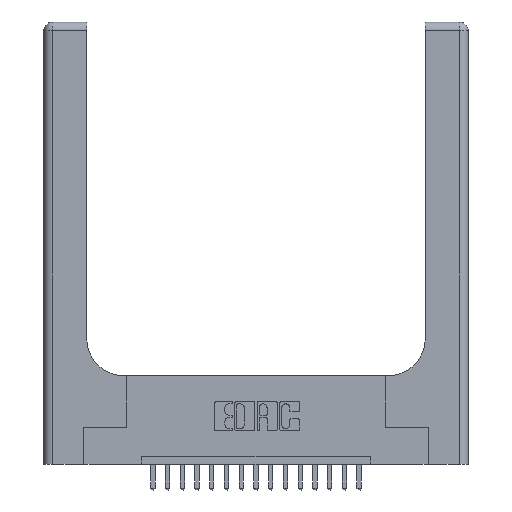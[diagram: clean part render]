
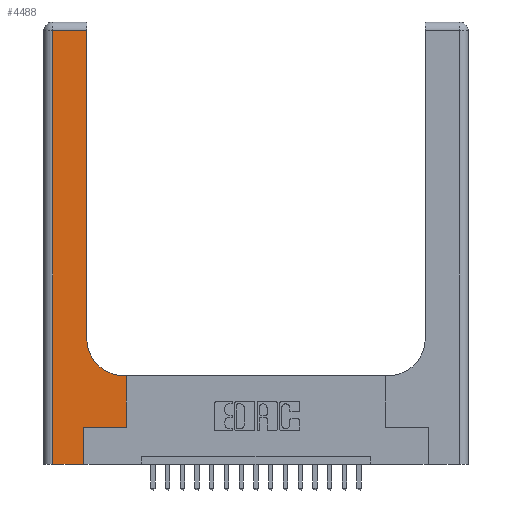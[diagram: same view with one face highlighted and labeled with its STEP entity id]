
A CAD part, top view. The second image highlights one B-rep face of the part: STEP entity #4488.
In plain terms, the highlighted planar face has unit normal (0, 0, 1).
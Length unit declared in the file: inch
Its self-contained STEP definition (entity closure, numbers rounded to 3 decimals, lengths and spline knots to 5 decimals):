
#148 = VECTOR ( 'NONE', #15924, 39.37008 ) ;
#211 = EDGE_CURVE ( 'NONE', #18725, #6965, #633, .T. ) ;
#633 = LINE ( 'NONE', #6570, #148 ) ;
#1206 = VERTEX_POINT ( 'NONE', #12824 ) ;
#1649 = VECTOR ( 'NONE', #11076, 39.37008 ) ;
#2056 = VECTOR ( 'NONE', #4676, 39.37008 ) ;
#2219 = EDGE_CURVE ( 'NONE', #10617, #5657, #18278, .T. ) ;
#2421 = CARTESIAN_POINT ( 'NONE',  ( 0.06, 0., 0.37 ) ) ;
#2588 = EDGE_CURVE ( 'NONE', #5657, #9849, #15346, .T. ) ;
#2597 = LINE ( 'NONE', #2917, #17723 ) ;
#2634 = VECTOR ( 'NONE', #16668, 39.37008 ) ;
#2917 = CARTESIAN_POINT ( 'NONE',  ( 0.2915, 0.6, 0.37 ) ) ;
#3111 = CARTESIAN_POINT ( 'NONE',  ( 0.269, 0., 0.37 ) ) ;
#3171 = DIRECTION ( 'NONE',  ( 0., 1., 0. ) ) ;
#3302 = EDGE_CURVE ( 'NONE', #10700, #18588, #15554, .T. ) ;
#3770 = LINE ( 'NONE', #3111, #2056 ) ;
#4225 = CARTESIAN_POINT ( 'NONE',  ( 0.269, 0., 0.37 ) ) ;
#4488 = ADVANCED_FACE ( 'NONE', ( #12314 ), #6179, .F. ) ;
#4625 = AXIS2_PLACEMENT_3D ( 'NONE', #11066, #9435, #5221 ) ;
#4671 = CARTESIAN_POINT ( 'NONE',  ( 0.5585, 0.6, 0.37 ) ) ;
#4676 = DIRECTION ( 'NONE',  ( 0., 1., 0. ) ) ;
#5146 = VERTEX_POINT ( 'NONE', #10031 ) ;
#5206 = ORIENTED_EDGE ( 'NONE', *, *, #19410, .T. ) ;
#5221 = DIRECTION ( 'NONE',  ( -1., 0., 0. ) ) ;
#5657 = VERTEX_POINT ( 'NONE', #7869 ) ;
#6179 = PLANE ( 'NONE',  #4625 ) ;
#6570 = CARTESIAN_POINT ( 'NONE',  ( 0., 2.94, 0.37 ) ) ;
#6953 = DIRECTION ( 'NONE',  ( 0., 1., 0. ) ) ;
#6965 = VERTEX_POINT ( 'NONE', #12682 ) ;
#7240 = VECTOR ( 'NONE', #10595, 39.37008 ) ;
#7242 = DIRECTION ( 'NONE',  ( 1., 0., 0. ) ) ;
#7333 = ORIENTED_EDGE ( 'NONE', *, *, #15643, .T. ) ;
#7588 = CIRCLE ( 'NONE', #10735, 0.25 ) ;
#7869 = CARTESIAN_POINT ( 'NONE',  ( 0.5585, 0.25, 0.37 ) ) ;
#7982 = DIRECTION ( 'NONE',  ( -1., 0., 0. ) ) ;
#8212 = CARTESIAN_POINT ( 'NONE',  ( 0.06, 3., 0.37 ) ) ;
#8257 = EDGE_CURVE ( 'NONE', #9849, #1206, #2597, .T. ) ;
#8568 = VECTOR ( 'NONE', #3171, 39.37008 ) ;
#9435 = DIRECTION ( 'NONE',  ( 0., 0., -1. ) ) ;
#9482 = CARTESIAN_POINT ( 'NONE',  ( 0.2915, 3., 0.37 ) ) ;
#9849 = VERTEX_POINT ( 'NONE', #4671 ) ;
#10031 = CARTESIAN_POINT ( 'NONE',  ( 0.2915, 0.85, 0.37 ) ) ;
#10049 = ORIENTED_EDGE ( 'NONE', *, *, #12741, .T. ) ;
#10530 = CARTESIAN_POINT ( 'NONE',  ( 0.2915, 2.94, 0.37 ) ) ;
#10595 = DIRECTION ( 'NONE',  ( 1., 0., 0. ) ) ;
#10617 = VERTEX_POINT ( 'NONE', #12881 ) ;
#10700 = VERTEX_POINT ( 'NONE', #2421 ) ;
#10735 = AXIS2_PLACEMENT_3D ( 'NONE', #16594, #19798, #7242 ) ;
#11066 = CARTESIAN_POINT ( 'NONE',  ( 0., 3., 0.37 ) ) ;
#11076 = DIRECTION ( 'NONE',  ( 0., -1., 0. ) ) ;
#12314 = FACE_OUTER_BOUND ( 'NONE', #19108, .T. ) ;
#12682 = CARTESIAN_POINT ( 'NONE',  ( 0.06, 2.94, 0.37 ) ) ;
#12741 = EDGE_CURVE ( 'NONE', #1206, #5146, #7588, .T. ) ;
#12824 = CARTESIAN_POINT ( 'NONE',  ( 0.5415, 0.6, 0.37 ) ) ;
#12881 = CARTESIAN_POINT ( 'NONE',  ( 0.269, 0.25, 0.37 ) ) ;
#13208 = ORIENTED_EDGE ( 'NONE', *, *, #8257, .T. ) ;
#13249 = ORIENTED_EDGE ( 'NONE', *, *, #2588, .T. ) ;
#13549 = ORIENTED_EDGE ( 'NONE', *, *, #17950, .T. ) ;
#13927 = CARTESIAN_POINT ( 'NONE',  ( 0., 0., 0.37 ) ) ;
#14221 = LINE ( 'NONE', #9482, #8568 ) ;
#14871 = VECTOR ( 'NONE', #6953, 39.37008 ) ;
#15346 = LINE ( 'NONE', #18906, #14871 ) ;
#15554 = LINE ( 'NONE', #13927, #7240 ) ;
#15643 = EDGE_CURVE ( 'NONE', #6965, #10700, #17238, .T. ) ;
#15924 = DIRECTION ( 'NONE',  ( -1., 0., 0. ) ) ;
#16594 = CARTESIAN_POINT ( 'NONE',  ( 0.5415, 0.85, 0.37 ) ) ;
#16668 = DIRECTION ( 'NONE',  ( 1., 0., 0. ) ) ;
#17238 = LINE ( 'NONE', #8212, #1649 ) ;
#17605 = ORIENTED_EDGE ( 'NONE', *, *, #3302, .T. ) ;
#17723 = VECTOR ( 'NONE', #7982, 39.37008 ) ;
#17950 = EDGE_CURVE ( 'NONE', #18588, #10617, #3770, .T. ) ;
#18278 = LINE ( 'NONE', #19526, #2634 ) ;
#18588 = VERTEX_POINT ( 'NONE', #4225 ) ;
#18725 = VERTEX_POINT ( 'NONE', #10530 ) ;
#18906 = CARTESIAN_POINT ( 'NONE',  ( 0.5585, 0.25, 0.37 ) ) ;
#19108 = EDGE_LOOP ( 'NONE', ( #5206, #19971, #7333, #17605, #13549, #20075, #13249, #13208, #10049 ) ) ;
#19410 = EDGE_CURVE ( 'NONE', #5146, #18725, #14221, .T. ) ;
#19526 = CARTESIAN_POINT ( 'NONE',  ( 0.269, 0.25, 0.37 ) ) ;
#19798 = DIRECTION ( 'NONE',  ( 0., 0., -1. ) ) ;
#19971 = ORIENTED_EDGE ( 'NONE', *, *, #211, .T. ) ;
#20075 = ORIENTED_EDGE ( 'NONE', *, *, #2219, .T. ) ;
